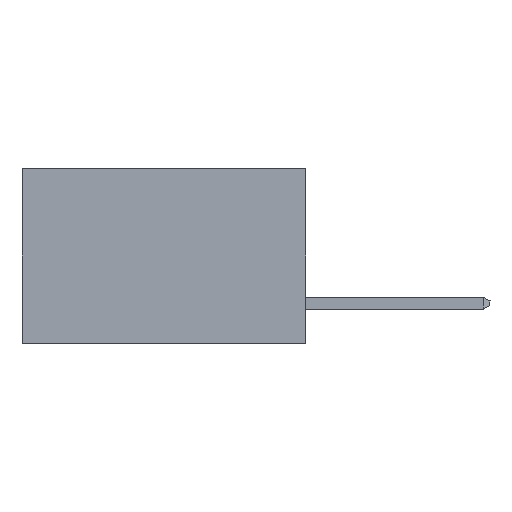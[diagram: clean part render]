
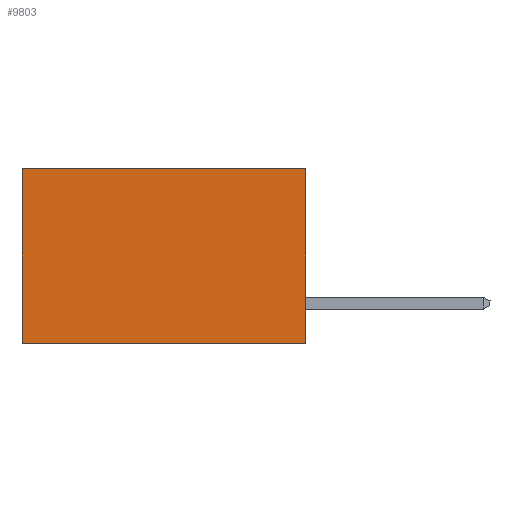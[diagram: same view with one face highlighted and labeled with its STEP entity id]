
A CAD part, left-side view. The second image highlights one B-rep face of the part: STEP entity #9803.
In plain terms, the highlighted planar face has unit normal (-1, 0, 0).
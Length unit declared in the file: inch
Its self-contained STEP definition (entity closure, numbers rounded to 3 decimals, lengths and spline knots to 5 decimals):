
#98 = CARTESIAN_POINT ( 'NONE',  ( 0.298, 0., 0. ) ) ;
#420 = VECTOR ( 'NONE', #9029, 39.37008 ) ;
#564 = LINE ( 'NONE', #1330, #420 ) ;
#661 = LINE ( 'NONE', #2337, #2951 ) ;
#1029 = DIRECTION ( 'NONE',  ( 1., 0., 0. ) ) ;
#1198 = CARTESIAN_POINT ( 'NONE',  ( 0.298, 0., 0. ) ) ;
#1330 = CARTESIAN_POINT ( 'NONE',  ( 0.298, 0., 0. ) ) ;
#1610 = ORIENTED_EDGE ( 'NONE', *, *, #10301, .T. ) ;
#1682 = VECTOR ( 'NONE', #2090, 39.37008 ) ;
#2000 = DIRECTION ( 'NONE',  ( 0., 0., -1. ) ) ;
#2090 = DIRECTION ( 'NONE',  ( 0., 1., 0. ) ) ;
#2335 = CARTESIAN_POINT ( 'NONE',  ( 0.298, 0., 0. ) ) ;
#2337 = CARTESIAN_POINT ( 'NONE',  ( 0.298, 0.6, 0. ) ) ;
#2428 = ORIENTED_EDGE ( 'NONE', *, *, #6378, .T. ) ;
#2951 = VECTOR ( 'NONE', #6576, 39.37008 ) ;
#3607 = AXIS2_PLACEMENT_3D ( 'NONE', #98, #1029, #2000 ) ;
#3726 = EDGE_CURVE ( 'NONE', #5508, #5849, #9488, .T. ) ;
#3834 = CARTESIAN_POINT ( 'NONE',  ( 0.298, 0., -0.37 ) ) ;
#3875 = EDGE_CURVE ( 'NONE', #9119, #5508, #564, .T. ) ;
#4402 = VERTEX_POINT ( 'NONE', #11344 ) ;
#5508 = VERTEX_POINT ( 'NONE', #3834 ) ;
#5771 = LINE ( 'NONE', #1198, #1682 ) ;
#5849 = VERTEX_POINT ( 'NONE', #10538 ) ;
#5964 = FACE_OUTER_BOUND ( 'NONE', #8155, .T. ) ;
#6378 = EDGE_CURVE ( 'NONE', #9119, #4402, #5771, .T. ) ;
#6576 = DIRECTION ( 'NONE',  ( 0., 0., -1. ) ) ;
#6859 = CARTESIAN_POINT ( 'NONE',  ( 0.298, 0., -0.37 ) ) ;
#8155 = EDGE_LOOP ( 'NONE', ( #1610, #9978, #8822, #2428 ) ) ;
#8822 = ORIENTED_EDGE ( 'NONE', *, *, #3875, .F. ) ;
#9029 = DIRECTION ( 'NONE',  ( 0., 0., -1. ) ) ;
#9119 = VERTEX_POINT ( 'NONE', #2335 ) ;
#9488 = LINE ( 'NONE', #6859, #12243 ) ;
#9703 = DIRECTION ( 'NONE',  ( 0., 1., 0. ) ) ;
#9803 = ADVANCED_FACE ( 'NONE', ( #5964 ), #10555, .F. ) ;
#9978 = ORIENTED_EDGE ( 'NONE', *, *, #3726, .F. ) ;
#10301 = EDGE_CURVE ( 'NONE', #4402, #5849, #661, .T. ) ;
#10538 = CARTESIAN_POINT ( 'NONE',  ( 0.298, 0.6, -0.37 ) ) ;
#10555 = PLANE ( 'NONE',  #3607 ) ;
#11344 = CARTESIAN_POINT ( 'NONE',  ( 0.298, 0.6, 0. ) ) ;
#12243 = VECTOR ( 'NONE', #9703, 39.37008 ) ;
